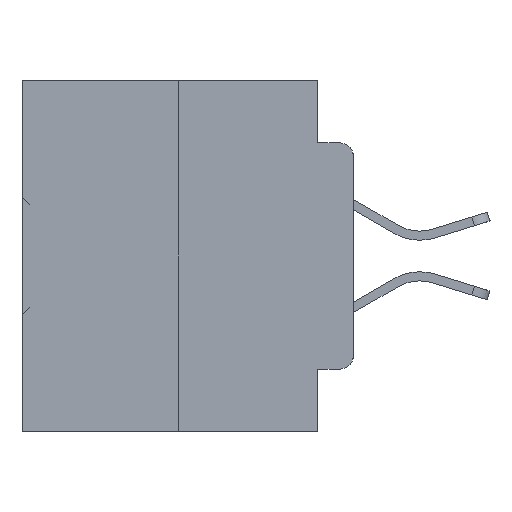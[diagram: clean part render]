
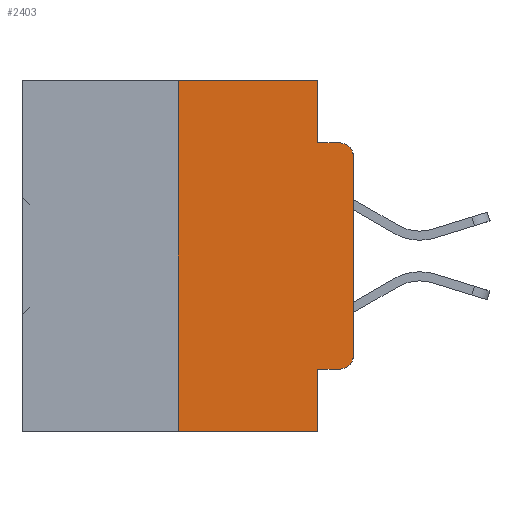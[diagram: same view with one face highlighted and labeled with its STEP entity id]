
A CAD part, left-side view. The second image highlights one B-rep face of the part: STEP entity #2403.
In plain terms, the highlighted planar face has unit normal (-1, 0, 0).
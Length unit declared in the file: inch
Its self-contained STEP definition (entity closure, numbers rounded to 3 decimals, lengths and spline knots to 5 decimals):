
#590 = ORIENTED_EDGE ( 'NONE', *, *, #23010, .T. ) ;
#2038 = CARTESIAN_POINT ( 'NONE',  ( 0., 0., 0. ) ) ;
#2403 = ADVANCED_FACE ( 'NONE', ( #33316 ), #13159, .F. ) ;
#2746 = LINE ( 'NONE', #2038, #14300 ) ;
#2929 = DIRECTION ( 'NONE',  ( 0., 0., 1. ) ) ;
#3122 = CARTESIAN_POINT ( 'NONE',  ( 0., 0.051, -0.0885 ) ) ;
#3882 = EDGE_LOOP ( 'NONE', ( #590, #34473, #26647, #19822, #28698, #27452, #37870, #22962, #14612, #11976 ) ) ;
#4625 = CARTESIAN_POINT ( 'NONE',  ( 0., 0.02, -0.0885 ) ) ;
#5669 = CARTESIAN_POINT ( 'NONE',  ( 0., 0.051, -0.0885 ) ) ;
#5916 = VERTEX_POINT ( 'NONE', #4625 ) ;
#6977 = VERTEX_POINT ( 'NONE', #5669 ) ;
#6994 = EDGE_CURVE ( 'NONE', #27857, #13800, #32166, .T. ) ;
#7900 = VECTOR ( 'NONE', #26530, 39.37008 ) ;
#8524 = CARTESIAN_POINT ( 'NONE',  ( 0., 0.473, -0.5 ) ) ;
#8567 = CARTESIAN_POINT ( 'NONE',  ( 0., 0.051, 0. ) ) ;
#8602 = DIRECTION ( 'NONE',  ( 0., -1., 0. ) ) ;
#8729 = VECTOR ( 'NONE', #17478, 39.37008 ) ;
#9089 = DIRECTION ( 'NONE',  ( 0., 0., -1. ) ) ;
#9134 = DIRECTION ( 'NONE',  ( 0., -1., 0. ) ) ;
#9326 = AXIS2_PLACEMENT_3D ( 'NONE', #21167, #34170, #19402 ) ;
#9508 = DIRECTION ( 'NONE',  ( 0., 0., -1. ) ) ;
#10122 = LINE ( 'NONE', #31024, #15177 ) ;
#11473 = LINE ( 'NONE', #14954, #12710 ) ;
#11525 = EDGE_CURVE ( 'NONE', #16133, #25836, #32196, .T. ) ;
#11976 = ORIENTED_EDGE ( 'NONE', *, *, #11525, .T. ) ;
#12462 = VECTOR ( 'NONE', #14493, 39.37008 ) ;
#12710 = VECTOR ( 'NONE', #8602, 39.37008 ) ;
#13159 = PLANE ( 'NONE',  #19077 ) ;
#13602 = VERTEX_POINT ( 'NONE', #8567 ) ;
#13800 = VERTEX_POINT ( 'NONE', #14918 ) ;
#14014 = CARTESIAN_POINT ( 'NONE',  ( 0., 0.051, 0. ) ) ;
#14059 = EDGE_CURVE ( 'NONE', #27857, #35559, #17190, .T. ) ;
#14300 = VECTOR ( 'NONE', #2929, 39.37008 ) ;
#14493 = DIRECTION ( 'NONE',  ( 0., -1., 0. ) ) ;
#14512 = CARTESIAN_POINT ( 'NONE',  ( 0., 0.02, -0.4115 ) ) ;
#14612 = ORIENTED_EDGE ( 'NONE', *, *, #27030, .T. ) ;
#14732 = CARTESIAN_POINT ( 'NONE',  ( 0., 0.25, 0. ) ) ;
#14918 = CARTESIAN_POINT ( 'NONE',  ( 0., 0.25, 0. ) ) ;
#14954 = CARTESIAN_POINT ( 'NONE',  ( 0., 0.473, 0. ) ) ;
#15046 = AXIS2_PLACEMENT_3D ( 'NONE', #29985, #35596, #9089 ) ;
#15177 = VECTOR ( 'NONE', #16111, 39.37008 ) ;
#16111 = DIRECTION ( 'NONE',  ( 0., 0., -1. ) ) ;
#16133 = VERTEX_POINT ( 'NONE', #14512 ) ;
#17190 = LINE ( 'NONE', #8524, #12462 ) ;
#17478 = DIRECTION ( 'NONE',  ( 0., 0., -1. ) ) ;
#18229 = CARTESIAN_POINT ( 'NONE',  ( 0., 0.051, -0.5 ) ) ;
#18231 = DIRECTION ( 'NONE',  ( 0., -1., 0. ) ) ;
#18368 = LINE ( 'NONE', #3122, #31110 ) ;
#19077 = AXIS2_PLACEMENT_3D ( 'NONE', #24958, #36780, #9508 ) ;
#19402 = DIRECTION ( 'NONE',  ( 0., 0., -1. ) ) ;
#19822 = ORIENTED_EDGE ( 'NONE', *, *, #34993, .F. ) ;
#21167 = CARTESIAN_POINT ( 'NONE',  ( 0., 0.02, -0.3915 ) ) ;
#22962 = ORIENTED_EDGE ( 'NONE', *, *, #34581, .F. ) ;
#23001 = CARTESIAN_POINT ( 'NONE',  ( 0., 0., -0.1085 ) ) ;
#23010 = EDGE_CURVE ( 'NONE', #25836, #23532, #2746, .T. ) ;
#23532 = VERTEX_POINT ( 'NONE', #23001 ) ;
#24486 = EDGE_CURVE ( 'NONE', #6977, #5916, #18368, .T. ) ;
#24891 = EDGE_CURVE ( 'NONE', #23532, #5916, #33599, .T. ) ;
#24958 = CARTESIAN_POINT ( 'NONE',  ( 0., 0.473, 0. ) ) ;
#25836 = VERTEX_POINT ( 'NONE', #35316 ) ;
#26530 = DIRECTION ( 'NONE',  ( 0., 0., 1. ) ) ;
#26647 = ORIENTED_EDGE ( 'NONE', *, *, #24486, .F. ) ;
#27030 = EDGE_CURVE ( 'NONE', #35178, #16133, #30083, .T. ) ;
#27452 = ORIENTED_EDGE ( 'NONE', *, *, #6994, .F. ) ;
#27857 = VERTEX_POINT ( 'NONE', #34909 ) ;
#28698 = ORIENTED_EDGE ( 'NONE', *, *, #29110, .F. ) ;
#29110 = EDGE_CURVE ( 'NONE', #13800, #13602, #11473, .T. ) ;
#29710 = CARTESIAN_POINT ( 'NONE',  ( 0., 0.051, -0.4115 ) ) ;
#29985 = CARTESIAN_POINT ( 'NONE',  ( 0., 0.02, -0.1085 ) ) ;
#29998 = VECTOR ( 'NONE', #18231, 39.37008 ) ;
#30083 = LINE ( 'NONE', #29710, #29998 ) ;
#31024 = CARTESIAN_POINT ( 'NONE',  ( 0., 0.051, 0. ) ) ;
#31110 = VECTOR ( 'NONE', #9134, 39.37008 ) ;
#32166 = LINE ( 'NONE', #14732, #7900 ) ;
#32196 = CIRCLE ( 'NONE', #9326, 0.02 ) ;
#32360 = CARTESIAN_POINT ( 'NONE',  ( 0., 0.051, -0.4115 ) ) ;
#33316 = FACE_OUTER_BOUND ( 'NONE', #3882, .T. ) ;
#33599 = CIRCLE ( 'NONE', #15046, 0.02 ) ;
#34170 = DIRECTION ( 'NONE',  ( -1., 0., 0. ) ) ;
#34473 = ORIENTED_EDGE ( 'NONE', *, *, #24891, .T. ) ;
#34581 = EDGE_CURVE ( 'NONE', #35178, #35559, #37449, .T. ) ;
#34909 = CARTESIAN_POINT ( 'NONE',  ( 0., 0.25, -0.5 ) ) ;
#34993 = EDGE_CURVE ( 'NONE', #13602, #6977, #10122, .T. ) ;
#35178 = VERTEX_POINT ( 'NONE', #32360 ) ;
#35316 = CARTESIAN_POINT ( 'NONE',  ( 0., 0., -0.3915 ) ) ;
#35559 = VERTEX_POINT ( 'NONE', #18229 ) ;
#35596 = DIRECTION ( 'NONE',  ( -1., 0., 0. ) ) ;
#36780 = DIRECTION ( 'NONE',  ( 1., 0., 0. ) ) ;
#37449 = LINE ( 'NONE', #14014, #8729 ) ;
#37870 = ORIENTED_EDGE ( 'NONE', *, *, #14059, .T. ) ;
